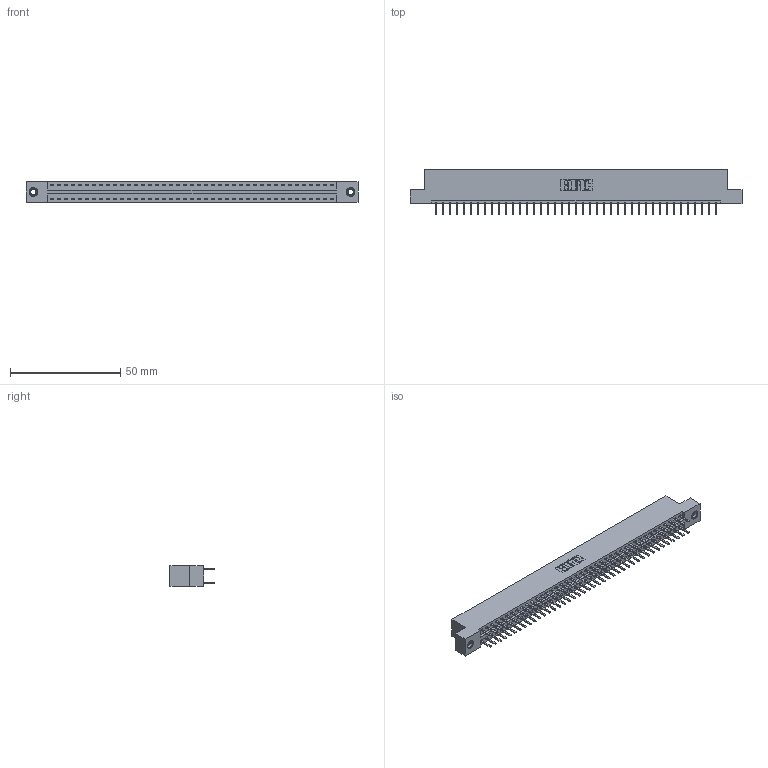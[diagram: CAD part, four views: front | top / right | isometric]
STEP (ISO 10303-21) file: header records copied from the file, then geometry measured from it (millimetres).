
FILE_DESCRIPTION (( 'STEP AP203' ), '1' );
FILE_NAME ('396-082-520-207.STEP', '2019-10-30T23:13:11', ( '' ), ( '' ), 'SwSTEP 2.0', 'SolidWorks 2016', '' );
FILE_SCHEMA (( 'CONFIG_CONTROL_DESIGN' ));
Length unit declared in the file: inch
Products named in the file (4): 346 Part_Flush Mounting Lugs - 0.156 Dia-TI; 396-082-520-207; 345-250-001_345-250-005-103; 345-292-001_345-293-120
Assembly tree (85 placements, depth 2):
  396-082-520-207
    346 Part_Flush Mounting Lugs - 0.156 Dia-TI
    345-292-001_345-293-120  x82
    345-250-001_345-250-005-103  x2
Bounding box: 150.75 x 20.02 x 9.4 mm (x, y, z)
Volume: 14642.6 mm3; surface area: 20060.8 mm2
Topology: 85 solids, 85 shells, 4774 faces, 13831 edges, 8994 vertices
Faces by surface type: plane 3142, cylinder 1616, cone 12, torus 4
Entity records: 28192 total; most frequent: CARTESIAN_POINT 4643, ORIENTED_EDGE 4558, DIRECTION 4157, EDGE_CURVE 2279, VECTOR 1959, LINE 1959, VERTEX_POINT 1512, AXIS2_PLACEMENT_3D 1099
